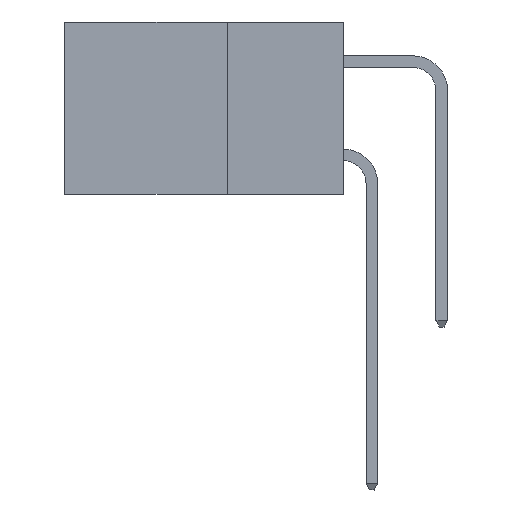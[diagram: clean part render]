
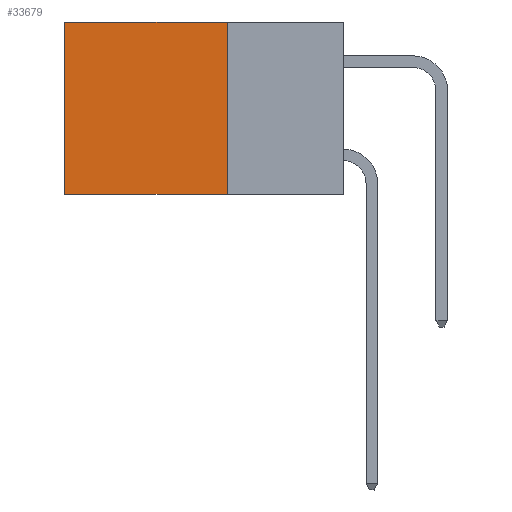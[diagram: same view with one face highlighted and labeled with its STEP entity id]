
A CAD part, left-side view. The second image highlights one B-rep face of the part: STEP entity #33679.
In plain terms, the highlighted planar face has unit normal (-1, 0, 0).
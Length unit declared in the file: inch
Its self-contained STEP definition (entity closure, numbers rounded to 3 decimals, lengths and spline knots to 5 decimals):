
#850 = LINE ( 'NONE', #30967, #13782 ) ;
#2544 = VERTEX_POINT ( 'NONE', #15507 ) ;
#3051 = VECTOR ( 'NONE', #17689, 39.37008 ) ;
#5153 = DIRECTION ( 'NONE',  ( 0., 0., -1. ) ) ;
#7315 = CARTESIAN_POINT ( 'NONE',  ( 0.298, 0.25, -0.37 ) ) ;
#7535 = DIRECTION ( 'NONE',  ( 0., 0., -1. ) ) ;
#8458 = ORIENTED_EDGE ( 'NONE', *, *, #22973, .T. ) ;
#8810 = CARTESIAN_POINT ( 'NONE',  ( 0.298, 0.6, -0.37 ) ) ;
#9092 = LINE ( 'NONE', #25488, #3051 ) ;
#9823 = ORIENTED_EDGE ( 'NONE', *, *, #14429, .T. ) ;
#9997 = DIRECTION ( 'NONE',  ( 0., 1., 0. ) ) ;
#11617 = VERTEX_POINT ( 'NONE', #16643 ) ;
#12652 = VERTEX_POINT ( 'NONE', #26467 ) ;
#12776 = PLANE ( 'NONE',  #24274 ) ;
#12815 = ORIENTED_EDGE ( 'NONE', *, *, #15830, .F. ) ;
#13782 = VECTOR ( 'NONE', #7535, 39.37008 ) ;
#14429 = EDGE_CURVE ( 'NONE', #12652, #11617, #17643, .T. ) ;
#15501 = EDGE_LOOP ( 'NONE', ( #8458, #12815, #21287, #9823 ) ) ;
#15507 = CARTESIAN_POINT ( 'NONE',  ( 0.298, 0.25, -0.37 ) ) ;
#15830 = EDGE_CURVE ( 'NONE', #2544, #19102, #15845, .T. ) ;
#15845 = LINE ( 'NONE', #7315, #22094 ) ;
#16643 = CARTESIAN_POINT ( 'NONE',  ( 0.298, 0.6, 0. ) ) ;
#17643 = LINE ( 'NONE', #22506, #30777 ) ;
#17689 = DIRECTION ( 'NONE',  ( 0., 0., -1. ) ) ;
#18106 = CARTESIAN_POINT ( 'NONE',  ( 0.298, 0.25, 0. ) ) ;
#19102 = VERTEX_POINT ( 'NONE', #8810 ) ;
#20770 = DIRECTION ( 'NONE',  ( 1., 0., 0. ) ) ;
#21287 = ORIENTED_EDGE ( 'NONE', *, *, #27039, .F. ) ;
#22094 = VECTOR ( 'NONE', #9997, 39.37008 ) ;
#22506 = CARTESIAN_POINT ( 'NONE',  ( 0.298, 0.25, 0. ) ) ;
#22973 = EDGE_CURVE ( 'NONE', #11617, #19102, #850, .T. ) ;
#24274 = AXIS2_PLACEMENT_3D ( 'NONE', #18106, #20770, #5153 ) ;
#25101 = DIRECTION ( 'NONE',  ( 0., 1., 0. ) ) ;
#25488 = CARTESIAN_POINT ( 'NONE',  ( 0.298, 0.25, 0. ) ) ;
#26467 = CARTESIAN_POINT ( 'NONE',  ( 0.298, 0.25, 0. ) ) ;
#27039 = EDGE_CURVE ( 'NONE', #12652, #2544, #9092, .T. ) ;
#30073 = FACE_OUTER_BOUND ( 'NONE', #15501, .T. ) ;
#30777 = VECTOR ( 'NONE', #25101, 39.37008 ) ;
#30967 = CARTESIAN_POINT ( 'NONE',  ( 0.298, 0.6, 0. ) ) ;
#33679 = ADVANCED_FACE ( 'NONE', ( #30073 ), #12776, .F. ) ;
